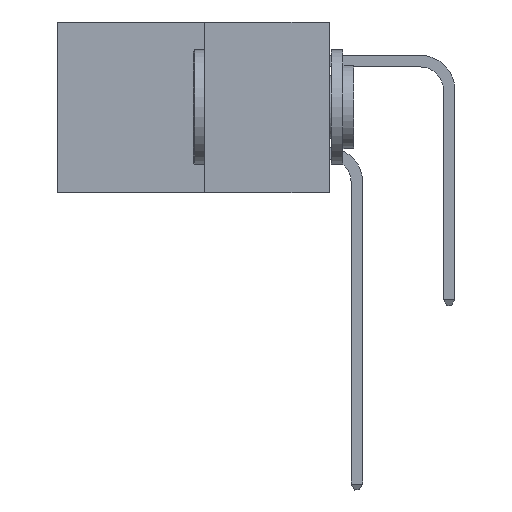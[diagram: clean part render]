
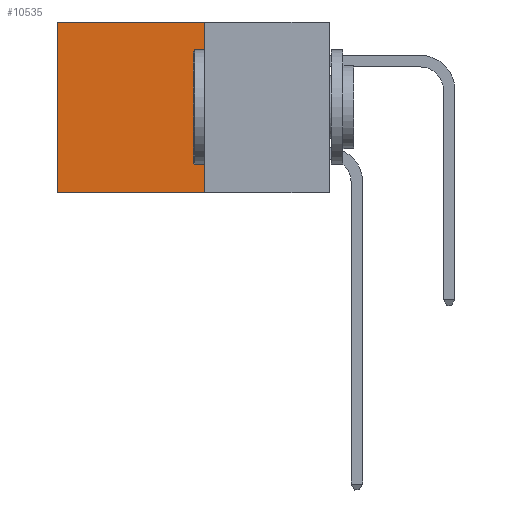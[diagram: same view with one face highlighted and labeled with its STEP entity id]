
A CAD part, left-side view. The second image highlights one B-rep face of the part: STEP entity #10535.
In plain terms, the highlighted planar face has unit normal (-1, 0, 0).
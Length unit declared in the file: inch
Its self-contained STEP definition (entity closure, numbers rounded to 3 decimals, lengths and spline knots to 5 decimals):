
#1372 = VERTEX_POINT ( 'NONE', #17545 ) ;
#1859 = ORIENTED_EDGE ( 'NONE', *, *, #8066, .F. ) ;
#2433 = VECTOR ( 'NONE', #10983, 39.37008 ) ;
#2778 = EDGE_CURVE ( 'NONE', #9591, #6893, #16272, .T. ) ;
#3369 = DIRECTION ( 'NONE',  ( 1., 0., 0. ) ) ;
#3930 = ORIENTED_EDGE ( 'NONE', *, *, #9655, .T. ) ;
#6244 = ORIENTED_EDGE ( 'NONE', *, *, #2778, .F. ) ;
#6516 = CARTESIAN_POINT ( 'NONE',  ( 0.277, 0.59, -0.37 ) ) ;
#6893 = VERTEX_POINT ( 'NONE', #6516 ) ;
#8066 = EDGE_CURVE ( 'NONE', #11129, #9591, #8549, .T. ) ;
#8314 = DIRECTION ( 'NONE',  ( 0., 0., -1. ) ) ;
#8549 = LINE ( 'NONE', #20709, #14066 ) ;
#9591 = VERTEX_POINT ( 'NONE', #16948 ) ;
#9655 = EDGE_CURVE ( 'NONE', #1372, #6893, #15970, .T. ) ;
#10535 = ADVANCED_FACE ( 'NONE', ( #17209 ), #15840, .F. ) ;
#10983 = DIRECTION ( 'NONE',  ( 0., 1., 0. ) ) ;
#11129 = VERTEX_POINT ( 'NONE', #21481 ) ;
#11407 = VECTOR ( 'NONE', #23260, 39.37008 ) ;
#13127 = CARTESIAN_POINT ( 'NONE',  ( 0.277, 0.59, -0.37 ) ) ;
#13154 = CARTESIAN_POINT ( 'NONE',  ( 0.277, 0.27, 0. ) ) ;
#13546 = LINE ( 'NONE', #13154, #2433 ) ;
#14066 = VECTOR ( 'NONE', #8314, 39.37008 ) ;
#14300 = EDGE_CURVE ( 'NONE', #11129, #1372, #13546, .T. ) ;
#15233 = DIRECTION ( 'NONE',  ( 0., 0., -1. ) ) ;
#15840 = PLANE ( 'NONE',  #26184 ) ;
#15970 = LINE ( 'NONE', #13127, #26209 ) ;
#16272 = LINE ( 'NONE', #23291, #11407 ) ;
#16948 = CARTESIAN_POINT ( 'NONE',  ( 0.277, 0.27, -0.37 ) ) ;
#17209 = FACE_OUTER_BOUND ( 'NONE', #20980, .T. ) ;
#17545 = CARTESIAN_POINT ( 'NONE',  ( 0.277, 0.59, 0. ) ) ;
#17936 = DIRECTION ( 'NONE',  ( 0., 0., -1. ) ) ;
#20709 = CARTESIAN_POINT ( 'NONE',  ( 0.277, 0.27, -0.37 ) ) ;
#20980 = EDGE_LOOP ( 'NONE', ( #3930, #6244, #1859, #24825 ) ) ;
#21481 = CARTESIAN_POINT ( 'NONE',  ( 0.277, 0.27, 0. ) ) ;
#21954 = CARTESIAN_POINT ( 'NONE',  ( 0.277, 0.27, -0.37 ) ) ;
#23260 = DIRECTION ( 'NONE',  ( 0., 1., 0. ) ) ;
#23291 = CARTESIAN_POINT ( 'NONE',  ( 0.277, 0.27, -0.37 ) ) ;
#24825 = ORIENTED_EDGE ( 'NONE', *, *, #14300, .T. ) ;
#26184 = AXIS2_PLACEMENT_3D ( 'NONE', #21954, #3369, #17936 ) ;
#26209 = VECTOR ( 'NONE', #15233, 39.37008 ) ;
